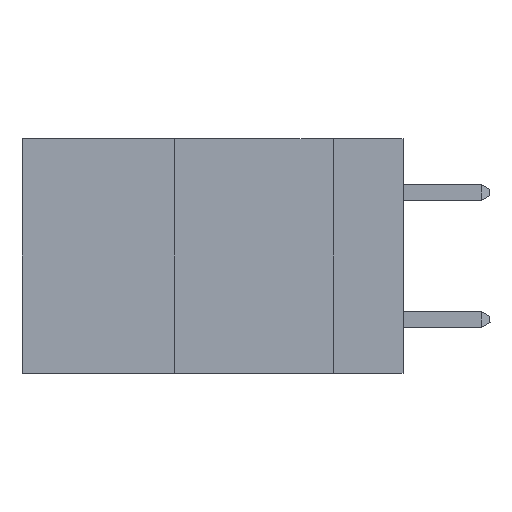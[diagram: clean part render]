
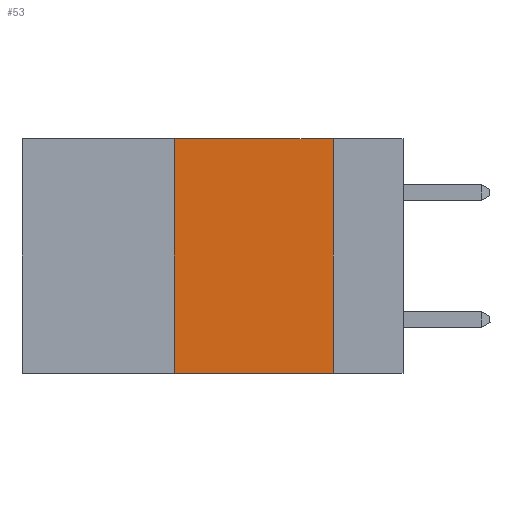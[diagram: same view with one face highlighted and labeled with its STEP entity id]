
A CAD part, left-side view. The second image highlights one B-rep face of the part: STEP entity #53.
In plain terms, the highlighted planar face has unit normal (-1, 0, 0).
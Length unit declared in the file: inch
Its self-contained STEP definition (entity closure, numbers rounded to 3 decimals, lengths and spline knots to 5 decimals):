
#53 = ADVANCED_FACE ( 'NONE', ( #29897 ), #22526, .F. ) ;
#1010 = VERTEX_POINT ( 'NONE', #10224 ) ;
#2229 = CARTESIAN_POINT ( 'NONE',  ( 0., 0.11, -0.37 ) ) ;
#4335 = DIRECTION ( 'NONE',  ( 0., 0., -1. ) ) ;
#4790 = CARTESIAN_POINT ( 'NONE',  ( 0., 0.36, 0. ) ) ;
#4979 = VECTOR ( 'NONE', #6467, 39.37008 ) ;
#5769 = AXIS2_PLACEMENT_3D ( 'NONE', #15658, #10956, #4335 ) ;
#5933 = EDGE_LOOP ( 'NONE', ( #15278, #17877, #7020, #27301 ) ) ;
#6467 = DIRECTION ( 'NONE',  ( 0., 0., 1. ) ) ;
#7020 = ORIENTED_EDGE ( 'NONE', *, *, #20659, .F. ) ;
#7835 = LINE ( 'NONE', #10329, #27103 ) ;
#7908 = VECTOR ( 'NONE', #25094, 39.37008 ) ;
#9990 = CARTESIAN_POINT ( 'NONE',  ( 0., 0.36, -0.37 ) ) ;
#10224 = CARTESIAN_POINT ( 'NONE',  ( 0., 0.11, 0. ) ) ;
#10329 = CARTESIAN_POINT ( 'NONE',  ( 0., 0.6, -0.37 ) ) ;
#10956 = DIRECTION ( 'NONE',  ( 1., 0., 0. ) ) ;
#11336 = LINE ( 'NONE', #18851, #4979 ) ;
#11906 = VERTEX_POINT ( 'NONE', #9990 ) ;
#12889 = LINE ( 'NONE', #13514, #7908 ) ;
#13514 = CARTESIAN_POINT ( 'NONE',  ( 0., 0.6, 0. ) ) ;
#15278 = ORIENTED_EDGE ( 'NONE', *, *, #23750, .F. ) ;
#15658 = CARTESIAN_POINT ( 'NONE',  ( 0., 0.6, 0. ) ) ;
#17877 = ORIENTED_EDGE ( 'NONE', *, *, #20567, .F. ) ;
#18851 = CARTESIAN_POINT ( 'NONE',  ( 0., 0.36, 0. ) ) ;
#20365 = DIRECTION ( 'NONE',  ( 0., 0., -1. ) ) ;
#20567 = EDGE_CURVE ( 'NONE', #24789, #1010, #12889, .T. ) ;
#20659 = EDGE_CURVE ( 'NONE', #11906, #24789, #11336, .T. ) ;
#21175 = VERTEX_POINT ( 'NONE', #2229 ) ;
#22526 = PLANE ( 'NONE',  #5769 ) ;
#22700 = CARTESIAN_POINT ( 'NONE',  ( 0., 0.11, 0. ) ) ;
#23004 = LINE ( 'NONE', #22700, #26524 ) ;
#23750 = EDGE_CURVE ( 'NONE', #1010, #21175, #23004, .T. ) ;
#24789 = VERTEX_POINT ( 'NONE', #4790 ) ;
#25094 = DIRECTION ( 'NONE',  ( 0., -1., 0. ) ) ;
#26524 = VECTOR ( 'NONE', #20365, 39.37008 ) ;
#27103 = VECTOR ( 'NONE', #28958, 39.37008 ) ;
#27301 = ORIENTED_EDGE ( 'NONE', *, *, #27411, .T. ) ;
#27411 = EDGE_CURVE ( 'NONE', #11906, #21175, #7835, .T. ) ;
#28958 = DIRECTION ( 'NONE',  ( 0., -1., 0. ) ) ;
#29897 = FACE_OUTER_BOUND ( 'NONE', #5933, .T. ) ;
